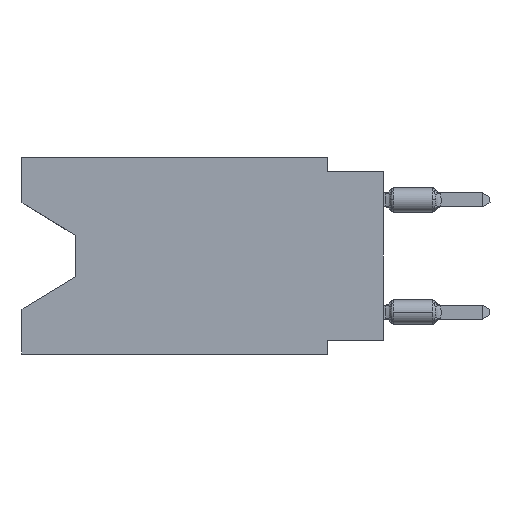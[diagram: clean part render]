
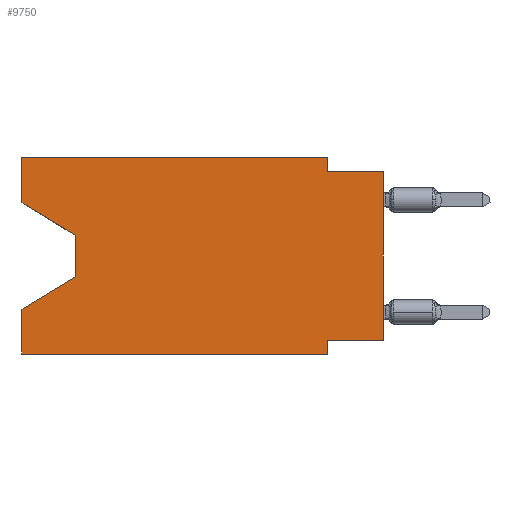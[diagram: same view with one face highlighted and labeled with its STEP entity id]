
A CAD part, left-side view. The second image highlights one B-rep face of the part: STEP entity #9750.
In plain terms, the highlighted planar face has unit normal (-1, 0, 0).
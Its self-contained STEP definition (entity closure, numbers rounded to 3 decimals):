
#65 = LINE ( 'NONE', #2706, #349 ) ;
#287 = EDGE_CURVE ( 'NONE', #14011, #6735, #5362, .T. ) ;
#349 = VECTOR ( 'NONE', #13060, 1000. ) ;
#555 = DIRECTION ( 'NONE',  ( 0., 0., 1. ) ) ;
#633 = VERTEX_POINT ( 'NONE', #3736 ) ;
#693 = DIRECTION ( 'NONE',  ( 0., -1., 0. ) ) ;
#806 = CARTESIAN_POINT ( 'NONE',  ( 0., 0., 0. ) ) ;
#915 = ORIENTED_EDGE ( 'NONE', *, *, #11792, .T. ) ;
#1019 = VERTEX_POINT ( 'NONE', #11448 ) ;
#1126 = ORIENTED_EDGE ( 'NONE', *, *, #8808, .T. ) ;
#1144 = CARTESIAN_POINT ( 'NONE',  ( 0., 13.97, -3.505 ) ) ;
#1389 = EDGE_CURVE ( 'NONE', #1019, #633, #12414, .T. ) ;
#1418 = EDGE_CURVE ( 'NONE', #5176, #16349, #8349, .T. ) ;
#1428 = DIRECTION ( 'NONE',  ( 0., -1., 0. ) ) ;
#1514 = CARTESIAN_POINT ( 'NONE',  ( 0., 16.383, -8.89 ) ) ;
#1521 = CARTESIAN_POINT ( 'NONE',  ( 0., 13.97, -3.505 ) ) ;
#2006 = CARTESIAN_POINT ( 'NONE',  ( 0., 2.54, 0. ) ) ;
#2074 = EDGE_CURVE ( 'NONE', #10190, #9745, #9243, .T. ) ;
#2108 = EDGE_CURVE ( 'NONE', #2388, #633, #6863, .T. ) ;
#2308 = VECTOR ( 'NONE', #8432, 1000. ) ;
#2316 = LINE ( 'NONE', #3241, #4420 ) ;
#2341 = DIRECTION ( 'NONE',  ( 0., 0., -1. ) ) ;
#2388 = VERTEX_POINT ( 'NONE', #11436 ) ;
#2631 = EDGE_CURVE ( 'NONE', #5489, #5176, #2316, .T. ) ;
#2706 = CARTESIAN_POINT ( 'NONE',  ( 0., 16.383, -2.038 ) ) ;
#2789 = DIRECTION ( 'NONE',  ( 0., -1., 0. ) ) ;
#2950 = CARTESIAN_POINT ( 'NONE',  ( 0., 0., -8.255 ) ) ;
#3241 = CARTESIAN_POINT ( 'NONE',  ( 0., 16.383, 0. ) ) ;
#3434 = CARTESIAN_POINT ( 'NONE',  ( 0., 0., -0.635 ) ) ;
#3736 = CARTESIAN_POINT ( 'NONE',  ( 0., 2.54, -8.89 ) ) ;
#3766 = LINE ( 'NONE', #1144, #4180 ) ;
#3835 = EDGE_CURVE ( 'NONE', #6922, #14011, #3766, .T. ) ;
#4122 = CARTESIAN_POINT ( 'NONE',  ( 0., 0., -8.255 ) ) ;
#4180 = VECTOR ( 'NONE', #2341, 1000. ) ;
#4420 = VECTOR ( 'NONE', #6141, 1000. ) ;
#4725 = EDGE_CURVE ( 'NONE', #2388, #6735, #6155, .T. ) ;
#5176 = VERTEX_POINT ( 'NONE', #14255 ) ;
#5324 = EDGE_CURVE ( 'NONE', #13487, #1019, #14667, .T. ) ;
#5362 = LINE ( 'NONE', #10545, #15203 ) ;
#5489 = VERTEX_POINT ( 'NONE', #15597 ) ;
#5588 = DIRECTION ( 'NONE',  ( 0., 1., 0. ) ) ;
#5707 = VECTOR ( 'NONE', #5588, 1000. ) ;
#5996 = VECTOR ( 'NONE', #16109, 1000. ) ;
#6069 = CARTESIAN_POINT ( 'NONE',  ( 0., 16.383, 0. ) ) ;
#6141 = DIRECTION ( 'NONE',  ( 0., 0., 1. ) ) ;
#6155 = LINE ( 'NONE', #6069, #8447 ) ;
#6156 = FACE_OUTER_BOUND ( 'NONE', #12860, .T. ) ;
#6735 = VERTEX_POINT ( 'NONE', #14258 ) ;
#6863 = LINE ( 'NONE', #1514, #13081 ) ;
#6922 = VERTEX_POINT ( 'NONE', #1521 ) ;
#7684 = VECTOR ( 'NONE', #2789, 1000. ) ;
#8349 = LINE ( 'NONE', #16157, #15865 ) ;
#8432 = DIRECTION ( 'NONE',  ( 0., 0., -1. ) ) ;
#8447 = VECTOR ( 'NONE', #14972, 1000. ) ;
#8477 = LINE ( 'NONE', #2006, #5996 ) ;
#8808 = EDGE_CURVE ( 'NONE', #13487, #9745, #9820, .T. ) ;
#8810 = ORIENTED_EDGE ( 'NONE', *, *, #2074, .F. ) ;
#8932 = ORIENTED_EDGE ( 'NONE', *, *, #1418, .F. ) ;
#9162 = CARTESIAN_POINT ( 'NONE',  ( 0., 0., -0.635 ) ) ;
#9205 = CARTESIAN_POINT ( 'NONE',  ( 0., 2.54, 0. ) ) ;
#9243 = LINE ( 'NONE', #9162, #7684 ) ;
#9497 = ORIENTED_EDGE ( 'NONE', *, *, #14451, .F. ) ;
#9745 = VERTEX_POINT ( 'NONE', #3434 ) ;
#9750 = ADVANCED_FACE ( 'NONE', ( #6156 ), #11330, .F. ) ;
#9775 = ORIENTED_EDGE ( 'NONE', *, *, #2108, .T. ) ;
#9820 = LINE ( 'NONE', #806, #10180 ) ;
#10055 = DIRECTION ( 'NONE',  ( 0., 0., -1. ) ) ;
#10180 = VECTOR ( 'NONE', #555, 1000. ) ;
#10190 = VERTEX_POINT ( 'NONE', #16746 ) ;
#10545 = CARTESIAN_POINT ( 'NONE',  ( 0., 13.97, -5.385 ) ) ;
#10972 = CARTESIAN_POINT ( 'NONE',  ( 0., 2.54, -8.89 ) ) ;
#11330 = PLANE ( 'NONE',  #15071 ) ;
#11436 = CARTESIAN_POINT ( 'NONE',  ( 0., 16.383, -8.89 ) ) ;
#11448 = CARTESIAN_POINT ( 'NONE',  ( 0., 2.54, -8.255 ) ) ;
#11792 = EDGE_CURVE ( 'NONE', #5489, #6922, #65, .T. ) ;
#12072 = ORIENTED_EDGE ( 'NONE', *, *, #2631, .F. ) ;
#12414 = LINE ( 'NONE', #10972, #2308 ) ;
#12860 = EDGE_LOOP ( 'NONE', ( #915, #15133, #15647, #15239, #9775, #13414, #14129, #1126, #8810, #9497, #8932, #12072 ) ) ;
#13060 = DIRECTION ( 'NONE',  ( 0., -0.855, -0.519 ) ) ;
#13081 = VECTOR ( 'NONE', #1428, 1000. ) ;
#13173 = DIRECTION ( 'NONE',  ( 0., 0.855, -0.519 ) ) ;
#13414 = ORIENTED_EDGE ( 'NONE', *, *, #1389, .F. ) ;
#13487 = VERTEX_POINT ( 'NONE', #4122 ) ;
#13778 = DIRECTION ( 'NONE',  ( 1., 0., 0. ) ) ;
#14011 = VERTEX_POINT ( 'NONE', #14701 ) ;
#14129 = ORIENTED_EDGE ( 'NONE', *, *, #5324, .F. ) ;
#14255 = CARTESIAN_POINT ( 'NONE',  ( 0., 16.383, 0. ) ) ;
#14258 = CARTESIAN_POINT ( 'NONE',  ( 0., 16.383, -6.852 ) ) ;
#14451 = EDGE_CURVE ( 'NONE', #16349, #10190, #8477, .T. ) ;
#14667 = LINE ( 'NONE', #2950, #5707 ) ;
#14701 = CARTESIAN_POINT ( 'NONE',  ( 0., 13.97, -5.385 ) ) ;
#14972 = DIRECTION ( 'NONE',  ( 0., 0., 1. ) ) ;
#15071 = AXIS2_PLACEMENT_3D ( 'NONE', #15321, #13778, #10055 ) ;
#15133 = ORIENTED_EDGE ( 'NONE', *, *, #3835, .T. ) ;
#15203 = VECTOR ( 'NONE', #13173, 1000. ) ;
#15239 = ORIENTED_EDGE ( 'NONE', *, *, #4725, .F. ) ;
#15321 = CARTESIAN_POINT ( 'NONE',  ( 0., 16.383, 0. ) ) ;
#15597 = CARTESIAN_POINT ( 'NONE',  ( 0., 16.383, -2.038 ) ) ;
#15647 = ORIENTED_EDGE ( 'NONE', *, *, #287, .T. ) ;
#15865 = VECTOR ( 'NONE', #693, 1000. ) ;
#16109 = DIRECTION ( 'NONE',  ( 0., 0., -1. ) ) ;
#16157 = CARTESIAN_POINT ( 'NONE',  ( 0., 16.383, 0. ) ) ;
#16349 = VERTEX_POINT ( 'NONE', #9205 ) ;
#16746 = CARTESIAN_POINT ( 'NONE',  ( 0., 2.54, -0.635 ) ) ;
